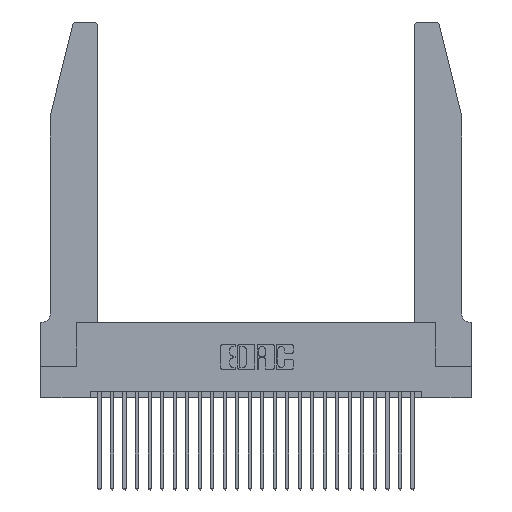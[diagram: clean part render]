
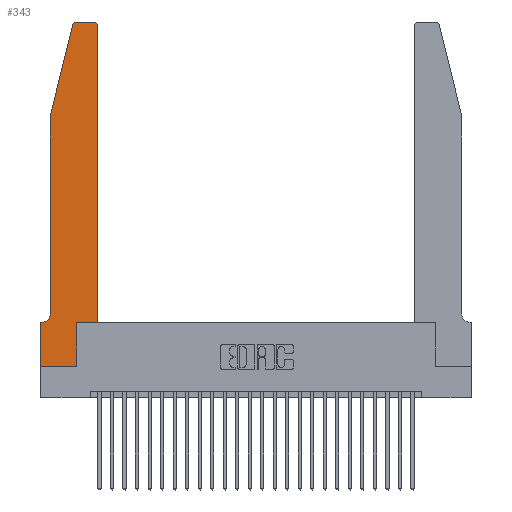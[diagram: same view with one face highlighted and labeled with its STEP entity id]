
A CAD part, top view. The second image highlights one B-rep face of the part: STEP entity #343.
In plain terms, the highlighted planar face has unit normal (0, 0, 1).
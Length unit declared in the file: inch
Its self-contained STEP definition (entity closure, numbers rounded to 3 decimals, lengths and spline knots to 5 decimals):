
#7 = DIRECTION ( 'NONE',  ( 1., 0., 0. ) ) ;
#188 = ORIENTED_EDGE ( 'NONE', *, *, #25524, .T. ) ;
#311 = DIRECTION ( 'NONE',  ( 1., 0., 0. ) ) ;
#343 = ADVANCED_FACE ( 'NONE', ( #11640 ), #24482, .T. ) ;
#832 = CARTESIAN_POINT ( 'NONE',  ( 0.2865, 0., 0.37 ) ) ;
#912 = EDGE_CURVE ( 'NONE', #18179, #10348, #26283, .T. ) ;
#914 = EDGE_LOOP ( 'NONE', ( #7545, #3968, #12942, #17838, #16535, #26984, #12602, #23077, #14243, #18477, #5931, #188 ) ) ;
#1030 = VERTEX_POINT ( 'NONE', #5333 ) ;
#1305 = EDGE_CURVE ( 'NONE', #22592, #1414, #18445, .T. ) ;
#1414 = VERTEX_POINT ( 'NONE', #1506 ) ;
#1466 = CARTESIAN_POINT ( 'NONE',  ( 0.4205, 2.75, 0.37 ) ) ;
#1506 = CARTESIAN_POINT ( 'NONE',  ( 0.2865, 0.35, 0.37 ) ) ;
#2174 = CARTESIAN_POINT ( 'NONE',  ( 0.4505, 0.35, 0.37 ) ) ;
#3098 = VECTOR ( 'NONE', #21280, 39.37008 ) ;
#3401 = EDGE_CURVE ( 'NONE', #26033, #22592, #8130, .T. ) ;
#3595 = CARTESIAN_POINT ( 'NONE',  ( 0.4505, 0.35, 0.37 ) ) ;
#3968 = ORIENTED_EDGE ( 'NONE', *, *, #17995, .T. ) ;
#4184 = DIRECTION ( 'NONE',  ( 0., 1., 0. ) ) ;
#4256 = CARTESIAN_POINT ( 'NONE',  ( 0.2865, 0.35, 0.37 ) ) ;
#4839 = DIRECTION ( 'NONE',  ( -1., 0., 0. ) ) ;
#5042 = VECTOR ( 'NONE', #7, 39.37008 ) ;
#5045 = CARTESIAN_POINT ( 'NONE',  ( 0., 0., 0.37 ) ) ;
#5093 = CARTESIAN_POINT ( 'NONE',  ( 0.0055, 0.42, 0.37 ) ) ;
#5186 = LINE ( 'NONE', #21355, #20721 ) ;
#5232 = AXIS2_PLACEMENT_3D ( 'NONE', #5093, #12396, #26084 ) ;
#5333 = CARTESIAN_POINT ( 'NONE',  ( 0., 0.35, 0.37 ) ) ;
#5931 = ORIENTED_EDGE ( 'NONE', *, *, #6527, .T. ) ;
#6283 = VECTOR ( 'NONE', #4839, 39.37008 ) ;
#6351 = DIRECTION ( 'NONE',  ( 0., 0., 1. ) ) ;
#6413 = CARTESIAN_POINT ( 'NONE',  ( 0.25487, 2.72718, 0.37 ) ) ;
#6527 = EDGE_CURVE ( 'NONE', #16635, #7869, #15208, .T. ) ;
#6539 = CARTESIAN_POINT ( 'NONE',  ( 0., 0., 0.37 ) ) ;
#6759 = CIRCLE ( 'NONE', #18840, 0.03 ) ;
#6773 = AXIS2_PLACEMENT_3D ( 'NONE', #21182, #8593, #23283 ) ;
#7109 = DIRECTION ( 'NONE',  ( -1., 0., 0. ) ) ;
#7220 = DIRECTION ( 'NONE',  ( 0., -1., 0. ) ) ;
#7502 = EDGE_CURVE ( 'NONE', #14997, #18179, #8192, .T. ) ;
#7545 = ORIENTED_EDGE ( 'NONE', *, *, #21244, .T. ) ;
#7869 = VERTEX_POINT ( 'NONE', #18868 ) ;
#8130 = LINE ( 'NONE', #6539, #3098 ) ;
#8192 = LINE ( 'NONE', #18239, #24277 ) ;
#8593 = DIRECTION ( 'NONE',  ( 0., 0., 1. ) ) ;
#8778 = DIRECTION ( 'NONE',  ( -0.239, -0.971, 0. ) ) ;
#9767 = EDGE_CURVE ( 'NONE', #1414, #16635, #16323, .T. ) ;
#10348 = VERTEX_POINT ( 'NONE', #21315 ) ;
#10870 = EDGE_CURVE ( 'NONE', #1030, #26033, #11690, .T. ) ;
#11374 = EDGE_CURVE ( 'NONE', #10348, #1030, #21865, .T. ) ;
#11416 = CARTESIAN_POINT ( 'NONE',  ( 0.0755, 0.35, 0.37 ) ) ;
#11586 = VECTOR ( 'NONE', #4184, 39.37008 ) ;
#11640 = FACE_OUTER_BOUND ( 'NONE', #914, .T. ) ;
#11690 = LINE ( 'NONE', #5045, #12988 ) ;
#12396 = DIRECTION ( 'NONE',  ( 0., 0., -1. ) ) ;
#12602 = ORIENTED_EDGE ( 'NONE', *, *, #10870, .T. ) ;
#12796 = DIRECTION ( 'NONE',  ( 0., 1., 0. ) ) ;
#12942 = ORIENTED_EDGE ( 'NONE', *, *, #25574, .T. ) ;
#12988 = VECTOR ( 'NONE', #7220, 39.37008 ) ;
#14114 = CARTESIAN_POINT ( 'NONE',  ( 0., 0.35, 0.37 ) ) ;
#14243 = ORIENTED_EDGE ( 'NONE', *, *, #1305, .T. ) ;
#14997 = VERTEX_POINT ( 'NONE', #26935 ) ;
#15208 = LINE ( 'NONE', #21132, #25632 ) ;
#16138 = DIRECTION ( 'NONE',  ( 0., -1., 0. ) ) ;
#16323 = LINE ( 'NONE', #2174, #5042 ) ;
#16535 = ORIENTED_EDGE ( 'NONE', *, *, #912, .T. ) ;
#16635 = VERTEX_POINT ( 'NONE', #3595 ) ;
#16856 = LINE ( 'NONE', #21736, #6283 ) ;
#17113 = CIRCLE ( 'NONE', #6773, 0.03 ) ;
#17327 = CARTESIAN_POINT ( 'NONE',  ( 0.0755, 0.42, 0.37 ) ) ;
#17838 = ORIENTED_EDGE ( 'NONE', *, *, #7502, .T. ) ;
#17995 = EDGE_CURVE ( 'NONE', #26069, #18703, #6759, .T. ) ;
#18179 = VERTEX_POINT ( 'NONE', #17327 ) ;
#18239 = CARTESIAN_POINT ( 'NONE',  ( 0.0755, 2., 0.37 ) ) ;
#18445 = LINE ( 'NONE', #4256, #11586 ) ;
#18477 = ORIENTED_EDGE ( 'NONE', *, *, #9767, .T. ) ;
#18703 = VERTEX_POINT ( 'NONE', #6413 ) ;
#18840 = AXIS2_PLACEMENT_3D ( 'NONE', #18981, #6351, #21093 ) ;
#18868 = CARTESIAN_POINT ( 'NONE',  ( 0.4505, 2.72, 0.37 ) ) ;
#18981 = CARTESIAN_POINT ( 'NONE',  ( 0.284, 2.72, 0.37 ) ) ;
#19248 = DIRECTION ( 'NONE',  ( 0., 0., 1. ) ) ;
#20721 = VECTOR ( 'NONE', #8778, 39.37008 ) ;
#20971 = CARTESIAN_POINT ( 'NONE',  ( 0., 0., 0.37 ) ) ;
#21093 = DIRECTION ( 'NONE',  ( 1., 0., 0. ) ) ;
#21132 = CARTESIAN_POINT ( 'NONE',  ( 0.4505, 0.35, 0.37 ) ) ;
#21182 = CARTESIAN_POINT ( 'NONE',  ( 0.4205, 2.72, 0.37 ) ) ;
#21225 = VECTOR ( 'NONE', #7109, 39.37008 ) ;
#21244 = EDGE_CURVE ( 'NONE', #23475, #26069, #16856, .T. ) ;
#21280 = DIRECTION ( 'NONE',  ( 1., 0., 0. ) ) ;
#21315 = CARTESIAN_POINT ( 'NONE',  ( 0.0055, 0.35, 0.37 ) ) ;
#21355 = CARTESIAN_POINT ( 'NONE',  ( 0.0755, 2., 0.37 ) ) ;
#21736 = CARTESIAN_POINT ( 'NONE',  ( 0.2605, 2.75, 0.37 ) ) ;
#21865 = LINE ( 'NONE', #11416, #21225 ) ;
#22592 = VERTEX_POINT ( 'NONE', #832 ) ;
#23077 = ORIENTED_EDGE ( 'NONE', *, *, #3401, .T. ) ;
#23166 = CARTESIAN_POINT ( 'NONE',  ( 0.284, 2.75, 0.37 ) ) ;
#23246 = AXIS2_PLACEMENT_3D ( 'NONE', #14114, #19248, #311 ) ;
#23283 = DIRECTION ( 'NONE',  ( 1., 0., 0. ) ) ;
#23475 = VERTEX_POINT ( 'NONE', #1466 ) ;
#24277 = VECTOR ( 'NONE', #16138, 39.37008 ) ;
#24482 = PLANE ( 'NONE',  #23246 ) ;
#25524 = EDGE_CURVE ( 'NONE', #7869, #23475, #17113, .T. ) ;
#25574 = EDGE_CURVE ( 'NONE', #18703, #14997, #5186, .T. ) ;
#25632 = VECTOR ( 'NONE', #12796, 39.37008 ) ;
#26033 = VERTEX_POINT ( 'NONE', #20971 ) ;
#26069 = VERTEX_POINT ( 'NONE', #23166 ) ;
#26084 = DIRECTION ( 'NONE',  ( -1., 0., 0. ) ) ;
#26283 = CIRCLE ( 'NONE', #5232, 0.07 ) ;
#26935 = CARTESIAN_POINT ( 'NONE',  ( 0.0755, 2., 0.37 ) ) ;
#26984 = ORIENTED_EDGE ( 'NONE', *, *, #11374, .T. ) ;
